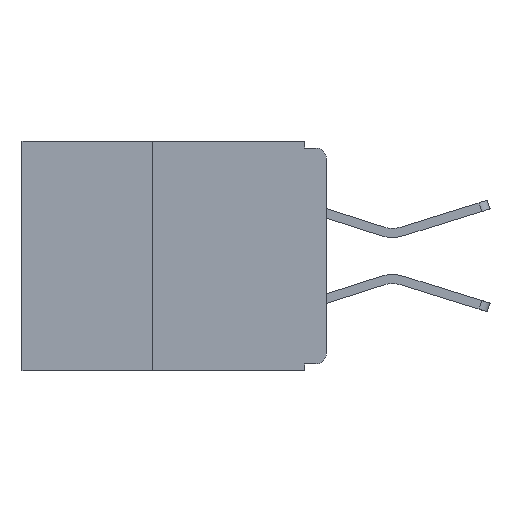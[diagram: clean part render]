
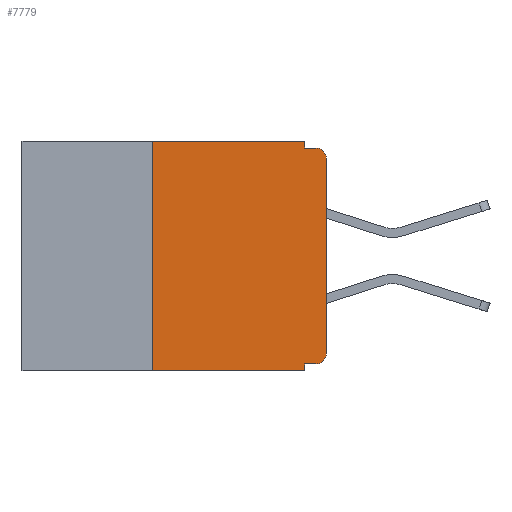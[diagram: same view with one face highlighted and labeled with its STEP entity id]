
A CAD part, left-side view. The second image highlights one B-rep face of the part: STEP entity #7779.
In plain terms, the highlighted planar face has unit normal (-1, 0, 0).
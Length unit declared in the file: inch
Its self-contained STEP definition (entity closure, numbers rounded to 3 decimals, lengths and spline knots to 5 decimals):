
#386 = DIRECTION ( 'NONE',  ( 0., -1., 0. ) ) ;
#408 = LINE ( 'NONE', #1509, #12921 ) ;
#472 = EDGE_CURVE ( 'NONE', #10290, #12130, #408, .T. ) ;
#493 = VECTOR ( 'NONE', #7021, 39.37008 ) ;
#603 = ORIENTED_EDGE ( 'NONE', *, *, #14874, .F. ) ;
#605 = CARTESIAN_POINT ( 'NONE',  ( 0., 0.031, 0. ) ) ;
#766 = VECTOR ( 'NONE', #386, 39.37008 ) ;
#776 = CARTESIAN_POINT ( 'NONE',  ( 0., 0.015, -0.32 ) ) ;
#896 = CARTESIAN_POINT ( 'NONE',  ( 0., 0.015, -0.025 ) ) ;
#940 = CARTESIAN_POINT ( 'NONE',  ( 0., 0.015, -0.305 ) ) ;
#1104 = VERTEX_POINT ( 'NONE', #10127 ) ;
#1200 = VERTEX_POINT ( 'NONE', #6225 ) ;
#1389 = DIRECTION ( 'NONE',  ( 0., 0., 1. ) ) ;
#1475 = EDGE_CURVE ( 'NONE', #4891, #12130, #5414, .T. ) ;
#1509 = CARTESIAN_POINT ( 'NONE',  ( 0., 0.031, -0.33 ) ) ;
#1570 = ORIENTED_EDGE ( 'NONE', *, *, #472, .F. ) ;
#1891 = AXIS2_PLACEMENT_3D ( 'NONE', #940, #9489, #2152 ) ;
#2107 = DIRECTION ( 'NONE',  ( 0., 0., -1. ) ) ;
#2152 = DIRECTION ( 'NONE',  ( 0., 0., -1. ) ) ;
#2326 = ORIENTED_EDGE ( 'NONE', *, *, #4931, .F. ) ;
#2484 = CARTESIAN_POINT ( 'NONE',  ( 0., 0.25, -0.33 ) ) ;
#2885 = LINE ( 'NONE', #7240, #15203 ) ;
#3179 = AXIS2_PLACEMENT_3D ( 'NONE', #896, #9447, #2107 ) ;
#3466 = VERTEX_POINT ( 'NONE', #11923 ) ;
#3543 = CARTESIAN_POINT ( 'NONE',  ( 0., 0.437, -0.33 ) ) ;
#3559 = DIRECTION ( 'NONE',  ( 0., -1., 0. ) ) ;
#3665 = ORIENTED_EDGE ( 'NONE', *, *, #4672, .F. ) ;
#3702 = EDGE_CURVE ( 'NONE', #15086, #1104, #4356, .T. ) ;
#3751 = LINE ( 'NONE', #5824, #493 ) ;
#3775 = CARTESIAN_POINT ( 'NONE',  ( 0., 0., -0.32 ) ) ;
#3832 = DIRECTION ( 'NONE',  ( 0., 1., 0. ) ) ;
#3950 = LINE ( 'NONE', #3775, #10038 ) ;
#4356 = LINE ( 'NONE', #7508, #13904 ) ;
#4417 = CARTESIAN_POINT ( 'NONE',  ( 0., 0., -0.305 ) ) ;
#4672 = EDGE_CURVE ( 'NONE', #4891, #1200, #3751, .T. ) ;
#4891 = VERTEX_POINT ( 'NONE', #2484 ) ;
#4931 = EDGE_CURVE ( 'NONE', #11893, #10290, #3950, .T. ) ;
#5312 = AXIS2_PLACEMENT_3D ( 'NONE', #13657, #14798, #7756 ) ;
#5414 = LINE ( 'NONE', #3543, #5805 ) ;
#5805 = VECTOR ( 'NONE', #3559, 39.37008 ) ;
#5824 = CARTESIAN_POINT ( 'NONE',  ( 0., 0.25, -0.33 ) ) ;
#6225 = CARTESIAN_POINT ( 'NONE',  ( 0., 0.25, 0. ) ) ;
#6563 = PLANE ( 'NONE',  #5312 ) ;
#7021 = DIRECTION ( 'NONE',  ( 0., 0., 1. ) ) ;
#7240 = CARTESIAN_POINT ( 'NONE',  ( 0., 0., -0.01 ) ) ;
#7274 = LINE ( 'NONE', #7743, #766 ) ;
#7319 = ORIENTED_EDGE ( 'NONE', *, *, #1475, .T. ) ;
#7508 = CARTESIAN_POINT ( 'NONE',  ( 0., 0., 0. ) ) ;
#7743 = CARTESIAN_POINT ( 'NONE',  ( 0., 0.437, 0. ) ) ;
#7756 = DIRECTION ( 'NONE',  ( 0., 0., -1. ) ) ;
#7779 = ADVANCED_FACE ( 'NONE', ( #13133 ), #6563, .F. ) ;
#8047 = EDGE_CURVE ( 'NONE', #11893, #15086, #9078, .T. ) ;
#8164 = EDGE_LOOP ( 'NONE', ( #9768, #13625, #12006, #603, #14521, #3665, #7319, #1570, #2326, #9235 ) ) ;
#8168 = CIRCLE ( 'NONE', #3179, 0.015 ) ;
#8475 = DIRECTION ( 'NONE',  ( 0., -1., 0. ) ) ;
#8953 = DIRECTION ( 'NONE',  ( 0., 0., -1. ) ) ;
#9078 = CIRCLE ( 'NONE', #1891, 0.015 ) ;
#9235 = ORIENTED_EDGE ( 'NONE', *, *, #8047, .T. ) ;
#9286 = VECTOR ( 'NONE', #8953, 39.37008 ) ;
#9447 = DIRECTION ( 'NONE',  ( -1., 0., 0. ) ) ;
#9461 = CARTESIAN_POINT ( 'NONE',  ( 0., 0.031, -0.01 ) ) ;
#9489 = DIRECTION ( 'NONE',  ( -1., 0., 0. ) ) ;
#9768 = ORIENTED_EDGE ( 'NONE', *, *, #3702, .T. ) ;
#10018 = VERTEX_POINT ( 'NONE', #605 ) ;
#10038 = VECTOR ( 'NONE', #3832, 39.37008 ) ;
#10075 = CARTESIAN_POINT ( 'NONE',  ( 0., 0.031, -0.33 ) ) ;
#10127 = CARTESIAN_POINT ( 'NONE',  ( 0., 0., -0.025 ) ) ;
#10264 = EDGE_CURVE ( 'NONE', #13667, #3466, #2885, .T. ) ;
#10290 = VERTEX_POINT ( 'NONE', #13222 ) ;
#11685 = EDGE_CURVE ( 'NONE', #1200, #10018, #7274, .T. ) ;
#11893 = VERTEX_POINT ( 'NONE', #776 ) ;
#11923 = CARTESIAN_POINT ( 'NONE',  ( 0., 0.015, -0.01 ) ) ;
#12006 = ORIENTED_EDGE ( 'NONE', *, *, #10264, .F. ) ;
#12130 = VERTEX_POINT ( 'NONE', #10075 ) ;
#12432 = LINE ( 'NONE', #14775, #9286 ) ;
#12833 = DIRECTION ( 'NONE',  ( 0., 0., -1. ) ) ;
#12921 = VECTOR ( 'NONE', #12833, 39.37008 ) ;
#13133 = FACE_OUTER_BOUND ( 'NONE', #8164, .T. ) ;
#13222 = CARTESIAN_POINT ( 'NONE',  ( 0., 0.031, -0.32 ) ) ;
#13625 = ORIENTED_EDGE ( 'NONE', *, *, #14180, .T. ) ;
#13657 = CARTESIAN_POINT ( 'NONE',  ( 0., 0.437, 0. ) ) ;
#13667 = VERTEX_POINT ( 'NONE', #9461 ) ;
#13904 = VECTOR ( 'NONE', #1389, 39.37008 ) ;
#14180 = EDGE_CURVE ( 'NONE', #1104, #3466, #8168, .T. ) ;
#14521 = ORIENTED_EDGE ( 'NONE', *, *, #11685, .F. ) ;
#14775 = CARTESIAN_POINT ( 'NONE',  ( 0., 0.031, 0. ) ) ;
#14798 = DIRECTION ( 'NONE',  ( 1., 0., 0. ) ) ;
#14874 = EDGE_CURVE ( 'NONE', #10018, #13667, #12432, .T. ) ;
#15086 = VERTEX_POINT ( 'NONE', #4417 ) ;
#15203 = VECTOR ( 'NONE', #8475, 39.37008 ) ;
